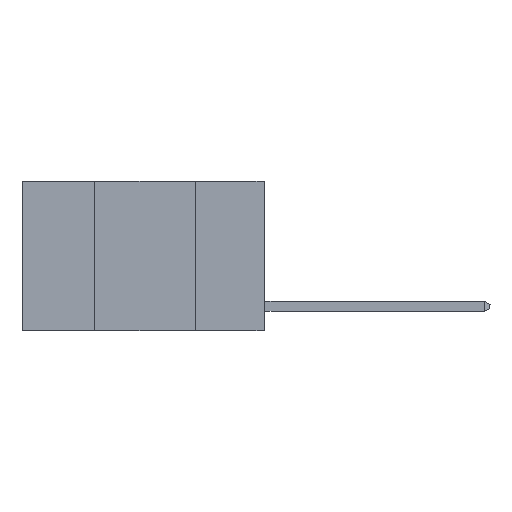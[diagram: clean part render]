
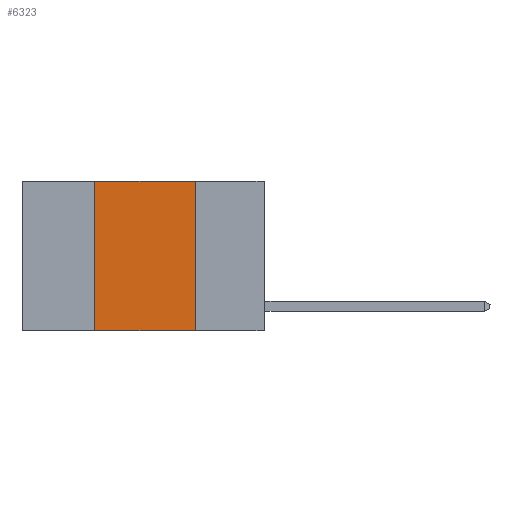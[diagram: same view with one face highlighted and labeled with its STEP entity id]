
A CAD part, left-side view. The second image highlights one B-rep face of the part: STEP entity #6323.
In plain terms, the highlighted planar face has unit normal (-1, 0, 0).
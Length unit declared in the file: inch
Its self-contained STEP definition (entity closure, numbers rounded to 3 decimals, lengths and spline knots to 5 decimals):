
#80 = EDGE_CURVE ( 'NONE', #17321, #10250, #8573, .T. ) ;
#115 = CARTESIAN_POINT ( 'NONE',  ( 0., 0.17, 0. ) ) ;
#1052 = CARTESIAN_POINT ( 'NONE',  ( 0., 0.17, -0.37 ) ) ;
#2010 = DIRECTION ( 'NONE',  ( 0., 0., -1. ) ) ;
#2493 = DIRECTION ( 'NONE',  ( 0., 0., 1. ) ) ;
#3035 = CARTESIAN_POINT ( 'NONE',  ( 0., 0.6, 0. ) ) ;
#3433 = CARTESIAN_POINT ( 'NONE',  ( 0., 0.17, 0. ) ) ;
#4489 = DIRECTION ( 'NONE',  ( 0., -1., 0. ) ) ;
#4898 = DIRECTION ( 'NONE',  ( 1., 0., 0. ) ) ;
#6323 = ADVANCED_FACE ( 'NONE', ( #8968 ), #21757, .F. ) ;
#6339 = DIRECTION ( 'NONE',  ( 0., -1., 0. ) ) ;
#6498 = CARTESIAN_POINT ( 'NONE',  ( 0., 0.6, 0. ) ) ;
#6657 = VERTEX_POINT ( 'NONE', #1052 ) ;
#7148 = AXIS2_PLACEMENT_3D ( 'NONE', #3035, #4898, #14044 ) ;
#7233 = ORIENTED_EDGE ( 'NONE', *, *, #80, .F. ) ;
#7268 = VERTEX_POINT ( 'NONE', #15050 ) ;
#8311 = CARTESIAN_POINT ( 'NONE',  ( 0., 0.6, -0.37 ) ) ;
#8573 = LINE ( 'NONE', #6498, #10351 ) ;
#8968 = FACE_OUTER_BOUND ( 'NONE', #19005, .T. ) ;
#9044 = ORIENTED_EDGE ( 'NONE', *, *, #22435, .F. ) ;
#10250 = VERTEX_POINT ( 'NONE', #3433 ) ;
#10351 = VECTOR ( 'NONE', #6339, 39.37008 ) ;
#10783 = LINE ( 'NONE', #22661, #23527 ) ;
#14044 = DIRECTION ( 'NONE',  ( 0., 0., -1. ) ) ;
#15050 = CARTESIAN_POINT ( 'NONE',  ( 0., 0.42, -0.37 ) ) ;
#16219 = LINE ( 'NONE', #115, #18529 ) ;
#16641 = LINE ( 'NONE', #8311, #22159 ) ;
#17321 = VERTEX_POINT ( 'NONE', #23396 ) ;
#18146 = ORIENTED_EDGE ( 'NONE', *, *, #19978, .T. ) ;
#18529 = VECTOR ( 'NONE', #2010, 39.37008 ) ;
#19005 = EDGE_LOOP ( 'NONE', ( #24000, #7233, #9044, #18146 ) ) ;
#19978 = EDGE_CURVE ( 'NONE', #7268, #6657, #16641, .T. ) ;
#21757 = PLANE ( 'NONE',  #7148 ) ;
#22159 = VECTOR ( 'NONE', #4489, 39.37008 ) ;
#22435 = EDGE_CURVE ( 'NONE', #7268, #17321, #10783, .T. ) ;
#22661 = CARTESIAN_POINT ( 'NONE',  ( 0., 0.42, 0. ) ) ;
#23396 = CARTESIAN_POINT ( 'NONE',  ( 0., 0.42, 0. ) ) ;
#23527 = VECTOR ( 'NONE', #2493, 39.37008 ) ;
#23990 = EDGE_CURVE ( 'NONE', #10250, #6657, #16219, .T. ) ;
#24000 = ORIENTED_EDGE ( 'NONE', *, *, #23990, .F. ) ;
